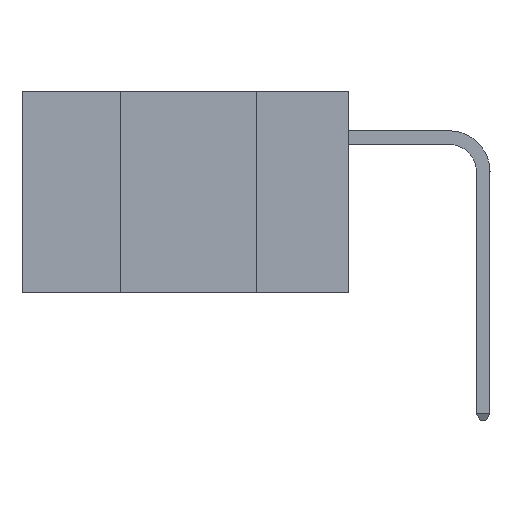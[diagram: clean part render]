
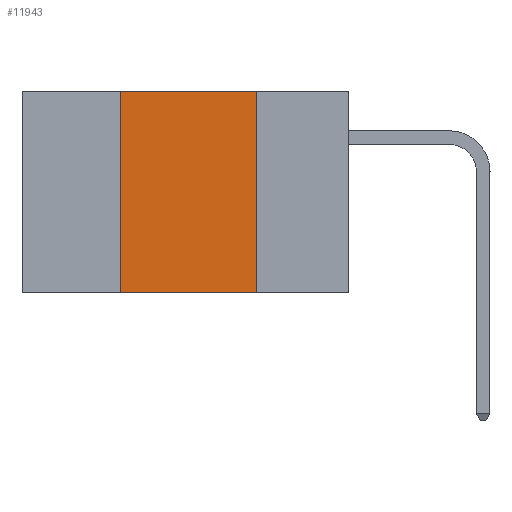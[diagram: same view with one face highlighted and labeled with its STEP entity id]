
A CAD part, left-side view. The second image highlights one B-rep face of the part: STEP entity #11943.
In plain terms, the highlighted planar face has unit normal (-1, 0, 0).
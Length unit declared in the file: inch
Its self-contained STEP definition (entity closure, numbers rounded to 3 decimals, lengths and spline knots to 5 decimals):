
#607 = CARTESIAN_POINT ( 'NONE',  ( 0., 0.6, -0.37 ) ) ;
#1095 = DIRECTION ( 'NONE',  ( 0., 0., -1. ) ) ;
#2871 = DIRECTION ( 'NONE',  ( 0., -1., 0. ) ) ;
#2945 = CARTESIAN_POINT ( 'NONE',  ( 0., 0.17, -0.37 ) ) ;
#3219 = CARTESIAN_POINT ( 'NONE',  ( 0., 0.6, 0. ) ) ;
#6177 = EDGE_CURVE ( 'NONE', #7074, #14969, #27248, .T. ) ;
#6503 = VERTEX_POINT ( 'NONE', #2945 ) ;
#6620 = EDGE_CURVE ( 'NONE', #7271, #6503, #22856, .T. ) ;
#7074 = VERTEX_POINT ( 'NONE', #10201 ) ;
#7271 = VERTEX_POINT ( 'NONE', #17995 ) ;
#7657 = VECTOR ( 'NONE', #2871, 39.37008 ) ;
#9436 = FACE_OUTER_BOUND ( 'NONE', #19318, .T. ) ;
#9546 = ORIENTED_EDGE ( 'NONE', *, *, #15686, .F. ) ;
#10201 = CARTESIAN_POINT ( 'NONE',  ( 0., 0.42, -0.37 ) ) ;
#11203 = LINE ( 'NONE', #607, #7657 ) ;
#11695 = PLANE ( 'NONE',  #18349 ) ;
#11943 = ADVANCED_FACE ( 'NONE', ( #9436 ), #11695, .F. ) ;
#13590 = CARTESIAN_POINT ( 'NONE',  ( 0., 0.6, 0. ) ) ;
#14491 = CARTESIAN_POINT ( 'NONE',  ( 0., 0.42, 0. ) ) ;
#14787 = CARTESIAN_POINT ( 'NONE',  ( 0., 0.17, 0. ) ) ;
#14969 = VERTEX_POINT ( 'NONE', #14491 ) ;
#15510 = ORIENTED_EDGE ( 'NONE', *, *, #6620, .F. ) ;
#15686 = EDGE_CURVE ( 'NONE', #14969, #7271, #22052, .T. ) ;
#16802 = CARTESIAN_POINT ( 'NONE',  ( 0., 0.42, 0. ) ) ;
#16836 = ORIENTED_EDGE ( 'NONE', *, *, #6177, .F. ) ;
#17995 = CARTESIAN_POINT ( 'NONE',  ( 0., 0.17, 0. ) ) ;
#18040 = VECTOR ( 'NONE', #24450, 39.37008 ) ;
#18349 = AXIS2_PLACEMENT_3D ( 'NONE', #3219, #20330, #1095 ) ;
#18914 = DIRECTION ( 'NONE',  ( 0., 0., 1. ) ) ;
#19318 = EDGE_LOOP ( 'NONE', ( #15510, #9546, #16836, #25868 ) ) ;
#20330 = DIRECTION ( 'NONE',  ( 1., 0., 0. ) ) ;
#22052 = LINE ( 'NONE', #13590, #18040 ) ;
#22856 = LINE ( 'NONE', #14787, #26760 ) ;
#24450 = DIRECTION ( 'NONE',  ( 0., -1., 0. ) ) ;
#24497 = EDGE_CURVE ( 'NONE', #7074, #6503, #11203, .T. ) ;
#25655 = DIRECTION ( 'NONE',  ( 0., 0., -1. ) ) ;
#25868 = ORIENTED_EDGE ( 'NONE', *, *, #24497, .T. ) ;
#26739 = VECTOR ( 'NONE', #18914, 39.37008 ) ;
#26760 = VECTOR ( 'NONE', #25655, 39.37008 ) ;
#27248 = LINE ( 'NONE', #16802, #26739 ) ;
